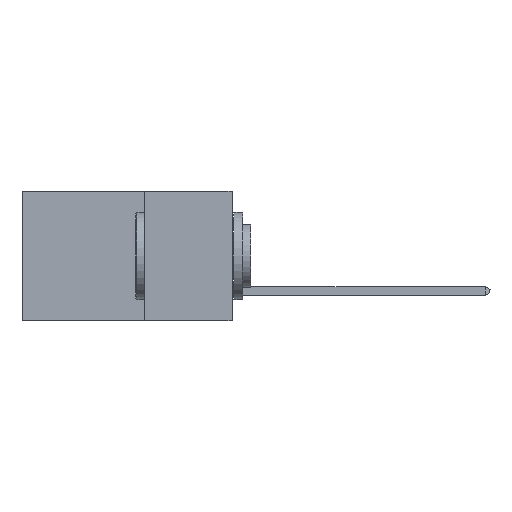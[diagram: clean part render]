
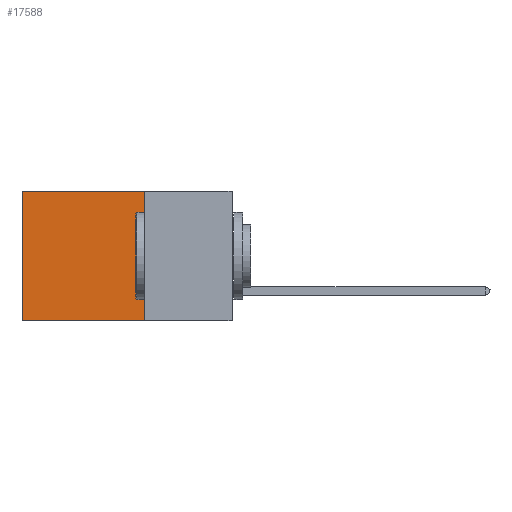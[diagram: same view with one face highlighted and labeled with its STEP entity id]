
A CAD part, left-side view. The second image highlights one B-rep face of the part: STEP entity #17588.
In plain terms, the highlighted planar face has unit normal (-1, 0, 0).
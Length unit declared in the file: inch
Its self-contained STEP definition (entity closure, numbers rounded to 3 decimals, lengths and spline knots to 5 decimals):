
#271 = CARTESIAN_POINT ( 'NONE',  ( 0.2875, 0.25, -0.37 ) ) ;
#2840 = EDGE_LOOP ( 'NONE', ( #23395, #20849, #7762, #11884 ) ) ;
#3164 = CARTESIAN_POINT ( 'NONE',  ( 0.2875, 0.25, 0. ) ) ;
#4403 = CARTESIAN_POINT ( 'NONE',  ( 0.2875, 0.25, 0. ) ) ;
#5112 = LINE ( 'NONE', #9102, #26709 ) ;
#5498 = EDGE_CURVE ( 'NONE', #17160, #9619, #14595, .T. ) ;
#7762 = ORIENTED_EDGE ( 'NONE', *, *, #7930, .F. ) ;
#7930 = EDGE_CURVE ( 'NONE', #13423, #24362, #11357, .T. ) ;
#8787 = FACE_OUTER_BOUND ( 'NONE', #2840, .T. ) ;
#9102 = CARTESIAN_POINT ( 'NONE',  ( 0.2875, 0.25, 0. ) ) ;
#9249 = DIRECTION ( 'NONE',  ( 0., 1., 0. ) ) ;
#9433 = LINE ( 'NONE', #271, #13024 ) ;
#9619 = VERTEX_POINT ( 'NONE', #22551 ) ;
#9794 = DIRECTION ( 'NONE',  ( 0., 0., -1. ) ) ;
#11105 = DIRECTION ( 'NONE',  ( 0., 0., -1. ) ) ;
#11357 = LINE ( 'NONE', #3164, #22476 ) ;
#11884 = ORIENTED_EDGE ( 'NONE', *, *, #19200, .T. ) ;
#11994 = VECTOR ( 'NONE', #11105, 39.37008 ) ;
#12889 = CARTESIAN_POINT ( 'NONE',  ( 0.2875, 0.6, 0. ) ) ;
#13024 = VECTOR ( 'NONE', #9249, 39.37008 ) ;
#13423 = VERTEX_POINT ( 'NONE', #4403 ) ;
#14595 = LINE ( 'NONE', #21662, #11994 ) ;
#16123 = PLANE ( 'NONE',  #17632 ) ;
#17160 = VERTEX_POINT ( 'NONE', #12889 ) ;
#17588 = ADVANCED_FACE ( 'NONE', ( #8787 ), #16123, .F. ) ;
#17632 = AXIS2_PLACEMENT_3D ( 'NONE', #20620, #24852, #22471 ) ;
#18148 = CARTESIAN_POINT ( 'NONE',  ( 0.2875, 0.25, -0.37 ) ) ;
#19200 = EDGE_CURVE ( 'NONE', #13423, #17160, #5112, .T. ) ;
#20620 = CARTESIAN_POINT ( 'NONE',  ( 0.2875, 0.25, 0. ) ) ;
#20849 = ORIENTED_EDGE ( 'NONE', *, *, #23147, .F. ) ;
#21662 = CARTESIAN_POINT ( 'NONE',  ( 0.2875, 0.6, 0. ) ) ;
#22471 = DIRECTION ( 'NONE',  ( 0., 0., -1. ) ) ;
#22476 = VECTOR ( 'NONE', #9794, 39.37008 ) ;
#22551 = CARTESIAN_POINT ( 'NONE',  ( 0.2875, 0.6, -0.37 ) ) ;
#23147 = EDGE_CURVE ( 'NONE', #24362, #9619, #9433, .T. ) ;
#23395 = ORIENTED_EDGE ( 'NONE', *, *, #5498, .T. ) ;
#24362 = VERTEX_POINT ( 'NONE', #18148 ) ;
#24852 = DIRECTION ( 'NONE',  ( 1., 0., 0. ) ) ;
#25811 = DIRECTION ( 'NONE',  ( 0., 1., 0. ) ) ;
#26709 = VECTOR ( 'NONE', #25811, 39.37008 ) ;
